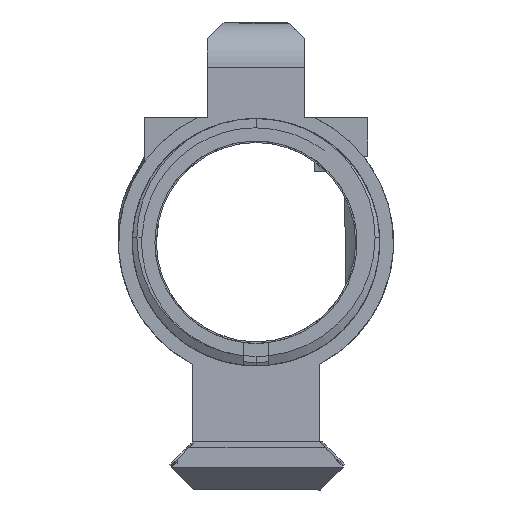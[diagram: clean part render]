
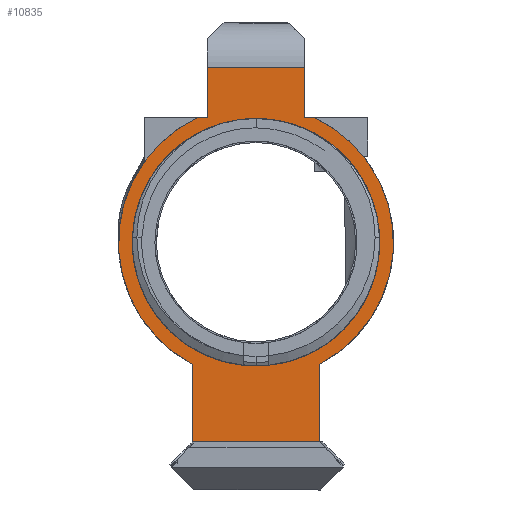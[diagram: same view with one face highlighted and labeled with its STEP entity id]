
A CAD part, left-side view. The second image highlights one B-rep face of the part: STEP entity #10835.
In plain terms, the highlighted planar face has unit normal (-1, 0, 0).
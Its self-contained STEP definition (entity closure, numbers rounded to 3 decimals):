
#91=FACE_BOUND('',#3710,.T.);
#1248=LINE('',#18209,#2219);
#1252=LINE('',#18217,#2223);
#1292=LINE('',#18703,#2263);
#1293=LINE('',#18705,#2264);
#1294=LINE('',#18707,#2265);
#1295=LINE('',#18709,#2266);
#1296=LINE('',#18710,#2267);
#1297=LINE('',#18712,#2268);
#1298=LINE('',#18714,#2269);
#1299=LINE('',#18715,#2270);
#2219=VECTOR('',#12538,1000.);
#2223=VECTOR('',#12542,1000.);
#2263=VECTOR('',#12638,1000.);
#2264=VECTOR('',#12639,1000.);
#2265=VECTOR('',#12640,10.);
#2266=VECTOR('',#12641,10.);
#2267=VECTOR('',#12642,1000.);
#2268=VECTOR('',#12643,1000.);
#2269=VECTOR('',#12644,1000.);
#2270=VECTOR('',#12645,1000.);
#3101=FACE_OUTER_BOUND('',#3709,.T.);
#3709=EDGE_LOOP('',(#8551,#8552,#8553,#8554,#8555,#8556,#8557,#8558,#8559,
#8560,#8561,#8562));
#3710=EDGE_LOOP('',(#8563));
#4046=CIRCLE('',#11315,17.621);
#4050=CIRCLE('',#11325,17.621);
#4055=CIRCLE('',#11333,14.891);
#4728=VERTEX_POINT('',#18206);
#4729=VERTEX_POINT('',#18208);
#4732=VERTEX_POINT('',#18214);
#4733=VERTEX_POINT('',#18216);
#4776=VERTEX_POINT('',#18415);
#4785=VERTEX_POINT('',#18450);
#4797=VERTEX_POINT('',#18702);
#4798=VERTEX_POINT('',#18704);
#4799=VERTEX_POINT('',#18706);
#4800=VERTEX_POINT('',#18708);
#4801=VERTEX_POINT('',#18711);
#4802=VERTEX_POINT('',#18713);
#4803=VERTEX_POINT('',#18716);
#6068=EDGE_CURVE('',#4728,#4729,#1248,.T.);
#6072=EDGE_CURVE('',#4732,#4733,#1252,.T.);
#6117=EDGE_CURVE('',#4776,#4728,#4046,.T.);
#6132=EDGE_CURVE('',#4733,#4785,#4050,.T.);
#6147=EDGE_CURVE('',#4776,#4797,#1292,.T.);
#6148=EDGE_CURVE('',#4797,#4798,#1293,.T.);
#6149=EDGE_CURVE('',#4798,#4799,#1294,.T.);
#6150=EDGE_CURVE('',#4800,#4799,#1295,.T.);
#6151=EDGE_CURVE('',#4785,#4800,#1296,.T.);
#6152=EDGE_CURVE('',#4732,#4801,#1297,.T.);
#6153=EDGE_CURVE('',#4801,#4802,#1298,.T.);
#6154=EDGE_CURVE('',#4802,#4729,#1299,.T.);
#6155=EDGE_CURVE('',#4803,#4803,#4055,.T.);
#8551=ORIENTED_EDGE('',*,*,#6068,.F.);
#8552=ORIENTED_EDGE('',*,*,#6117,.F.);
#8553=ORIENTED_EDGE('',*,*,#6147,.T.);
#8554=ORIENTED_EDGE('',*,*,#6148,.T.);
#8555=ORIENTED_EDGE('',*,*,#6149,.T.);
#8556=ORIENTED_EDGE('',*,*,#6150,.F.);
#8557=ORIENTED_EDGE('',*,*,#6151,.F.);
#8558=ORIENTED_EDGE('',*,*,#6132,.F.);
#8559=ORIENTED_EDGE('',*,*,#6072,.F.);
#8560=ORIENTED_EDGE('',*,*,#6152,.T.);
#8561=ORIENTED_EDGE('',*,*,#6153,.T.);
#8562=ORIENTED_EDGE('',*,*,#6154,.T.);
#8563=ORIENTED_EDGE('',*,*,#6155,.T.);
#10377=PLANE('',#11332);
#10835=ADVANCED_FACE('',(#3101,#91),#10377,.F.);
#11315=AXIS2_PLACEMENT_3D('',#18417,#12588,#12589);
#11325=AXIS2_PLACEMENT_3D('',#18451,#12617,#12618);
#11332=AXIS2_PLACEMENT_3D('',#18701,#12636,#12637);
#11333=AXIS2_PLACEMENT_3D('',#18717,#12646,#12647);
#12538=DIRECTION('',(0.,0.,-1.));
#12542=DIRECTION('',(0.,0.,-1.));
#12588=DIRECTION('center_axis',(1.,0.,0.));
#12589=DIRECTION('ref_axis',(0.,0.,1.));
#12617=DIRECTION('center_axis',(1.,0.,0.));
#12618=DIRECTION('ref_axis',(0.,0.,-1.));
#12636=DIRECTION('center_axis',(1.,0.,0.));
#12637=DIRECTION('ref_axis',(0.,1.,0.));
#12638=DIRECTION('',(0.,1.,0.));
#12639=DIRECTION('',(0.,0.,-1.));
#12640=DIRECTION('',(0.,-0.707,-0.707));
#12641=DIRECTION('',(0.,-0.707,0.707));
#12642=DIRECTION('',(0.,1.,0.));
#12643=DIRECTION('',(0.,-1.,0.));
#12644=DIRECTION('',(0.,0.,1.));
#12645=DIRECTION('',(0.,1.,0.));
#12646=DIRECTION('center_axis',(1.,0.,0.));
#12647=DIRECTION('ref_axis',(0.,0.,1.));
#18206=CARTESIAN_POINT('',(393.794,168.042,21.222));
#18208=CARTESIAN_POINT('',(393.794,168.042,20.063));
#18209=CARTESIAN_POINT('',(393.794,168.042,-1.067));
#18214=CARTESIAN_POINT('',(393.794,168.042,7.515));
#18216=CARTESIAN_POINT('',(393.794,168.042,6.355));
#18217=CARTESIAN_POINT('',(393.794,168.042,-1.067));
#18415=CARTESIAN_POINT('',(393.794,199.673,21.879));
#18417=CARTESIAN_POINT('Origin',(393.794,184.018,13.789));
#18450=CARTESIAN_POINT('',(393.794,199.673,5.699));
#18451=CARTESIAN_POINT('Origin',(393.794,184.018,13.789));
#18701=CARTESIAN_POINT('Origin',(393.794,161.692,-1.635));
#18702=CARTESIAN_POINT('',(393.794,209.594,21.879));
#18703=CARTESIAN_POINT('',(393.794,183.282,21.879));
#18704=CARTESIAN_POINT('',(393.794,209.594,5.769));
#18705=CARTESIAN_POINT('',(393.794,209.594,1.816));
#18706=CARTESIAN_POINT('',(393.794,209.542,5.717));
#18707=CARTESIAN_POINT('',(393.794,209.594,5.769));
#18708=CARTESIAN_POINT('',(393.794,209.56,5.699));
#18709=CARTESIAN_POINT('',(393.794,208.441,6.818));
#18710=CARTESIAN_POINT('',(393.794,183.282,5.699));
#18711=CARTESIAN_POINT('',(393.794,161.692,7.515));
#18712=CARTESIAN_POINT('',(393.794,159.838,7.515));
#18713=CARTESIAN_POINT('',(393.794,161.692,20.063));
#18714=CARTESIAN_POINT('',(393.794,161.692,7.515));
#18715=CARTESIAN_POINT('',(393.794,164.867,20.063));
#18716=CARTESIAN_POINT('',(393.794,184.018,-1.102));
#18717=CARTESIAN_POINT('Origin',(393.794,184.018,13.789));
